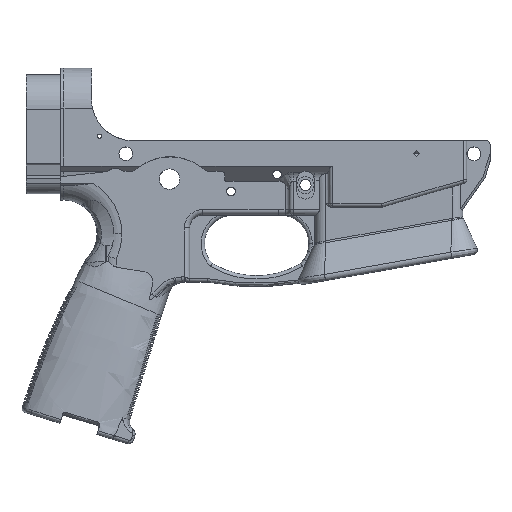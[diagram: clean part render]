
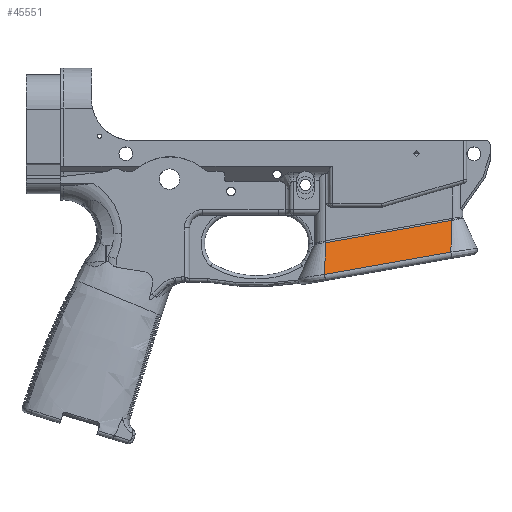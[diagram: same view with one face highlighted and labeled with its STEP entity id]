
A CAD part, top view. The second image highlights one B-rep face of the part: STEP entity #45551.
In plain terms, the highlighted planar face has unit normal (-0.074, 0.423, 0.903).
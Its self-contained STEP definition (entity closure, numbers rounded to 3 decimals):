
#2194 = ORIENTED_EDGE ( 'NONE', *, *, #14546, .F. ) ;
#3659 = DIRECTION ( 'NONE',  ( 0., -0.906, 0.424 ) ) ;
#3806 = ORIENTED_EDGE ( 'NONE', *, *, #65800, .T. ) ;
#4645 = DIRECTION ( 'NONE',  ( 0.035, 0.906, -0.421 ) ) ;
#5196 = LINE ( 'NONE', #72499, #58906 ) ;
#5670 = VERTEX_POINT ( 'NONE', #17099 ) ;
#6873 = DIRECTION ( 'NONE',  ( 0.035, 0.906, -0.421 ) ) ;
#9150 = EDGE_CURVE ( 'NONE', #17012, #65678, #25840, .T. ) ;
#14174 = CARTESIAN_POINT ( 'NONE',  ( -68.766, -41.045, 15.444 ) ) ;
#14546 = EDGE_CURVE ( 'NONE', #5670, #79381, #5196, .T. ) ;
#15368 = CARTESIAN_POINT ( 'NONE',  ( -10.222, -30.723, 15.444 ) ) ;
#16532 =( BOUNDED_CURVE ( )  B_SPLINE_CURVE ( 3, ( #21853, #48210, #55104, #68501 ),
 .UNSPECIFIED., .F., .F. ) 
 B_SPLINE_CURVE_WITH_KNOTS ( ( 4, 4 ),
 ( 3.059, 3.083 ),
 .UNSPECIFIED. ) 
 CURVE ( )  GEOMETRIC_REPRESENTATION_ITEM ( )  RATIONAL_B_SPLINE_CURVE ( ( 1., 1., 1., 1. ) ) 
 REPRESENTATION_ITEM ( '' )  );
#17012 = VERTEX_POINT ( 'NONE', #15368 ) ;
#17099 = CARTESIAN_POINT ( 'NONE',  ( -69.498, -55.858, 22.314 ) ) ;
#19955 = CARTESIAN_POINT ( 'NONE',  ( -10.789, -45.507, 22.314 ) ) ;
#21853 = CARTESIAN_POINT ( 'NONE',  ( -68.766, -41.045, 15.444 ) ) ;
#23500 = FACE_OUTER_BOUND ( 'NONE', #83841, .T. ) ;
#25840 = LINE ( 'NONE', #29450, #27250 ) ;
#27250 = VECTOR ( 'NONE', #82109, 1000. ) ;
#28656 = VECTOR ( 'NONE', #4645, 1000. ) ;
#29450 = CARTESIAN_POINT ( 'NONE',  ( -10.135, -30.707, 15.444 ) ) ;
#30112 = LINE ( 'NONE', #84055, #28656 ) ;
#33297 = ORIENTED_EDGE ( 'NONE', *, *, #33474, .T. ) ;
#33474 = EDGE_CURVE ( 'NONE', #65678, #79381, #16532, .T. ) ;
#42071 = DIRECTION ( 'NONE',  ( -0.075, 0.423, 0.903 ) ) ;
#44876 = DIRECTION ( 'NONE',  ( 0.985, 0.174, 0. ) ) ;
#45551 = ADVANCED_FACE ( 'NONE', ( #23500 ), #62386, .T. ) ;
#48210 = CARTESIAN_POINT ( 'NONE',  ( -68.821, -41.055, 15.444 ) ) ;
#54997 = EDGE_CURVE ( 'NONE', #5670, #58805, #70792, .T. ) ;
#55104 = CARTESIAN_POINT ( 'NONE',  ( -68.876, -41.063, 15.443 ) ) ;
#58248 = VECTOR ( 'NONE', #44876, 1000. ) ;
#58805 = VERTEX_POINT ( 'NONE', #19955 ) ;
#58906 = VECTOR ( 'NONE', #6873, 1000. ) ;
#62386 = PLANE ( 'NONE',  #81905 ) ;
#65678 = VERTEX_POINT ( 'NONE', #14174 ) ;
#65800 = EDGE_CURVE ( 'NONE', #58805, #17012, #30112, .T. ) ;
#68501 = CARTESIAN_POINT ( 'NONE',  ( -68.931, -41.07, 15.442 ) ) ;
#68740 = CARTESIAN_POINT ( 'NONE',  ( -68.931, -41.07, 15.442 ) ) ;
#70792 = LINE ( 'NONE', #76407, #58248 ) ;
#72238 = ORIENTED_EDGE ( 'NONE', *, *, #9150, .T. ) ;
#72499 = CARTESIAN_POINT ( 'NONE',  ( -68.915, -40.658, 15.25 ) ) ;
#76407 = CARTESIAN_POINT ( 'NONE',  ( -11.397, -45.614, 22.314 ) ) ;
#79381 = VERTEX_POINT ( 'NONE', #68740 ) ;
#81905 = AXIS2_PLACEMENT_3D ( 'NONE', #82224, #42071, #3659 ) ;
#82109 = DIRECTION ( 'NONE',  ( -0.985, -0.174, 0. ) ) ;
#82224 = CARTESIAN_POINT ( 'NONE',  ( -10.206, -30.306, 15.25 ) ) ;
#83061 = ORIENTED_EDGE ( 'NONE', *, *, #54997, .T. ) ;
#83841 = EDGE_LOOP ( 'NONE', ( #3806, #72238, #33297, #2194, #83061 ) ) ;
#84055 = CARTESIAN_POINT ( 'NONE',  ( -10.206, -30.306, 15.25 ) ) ;
